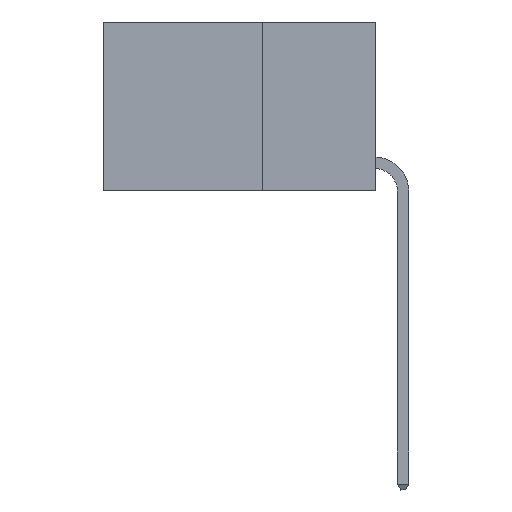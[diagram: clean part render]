
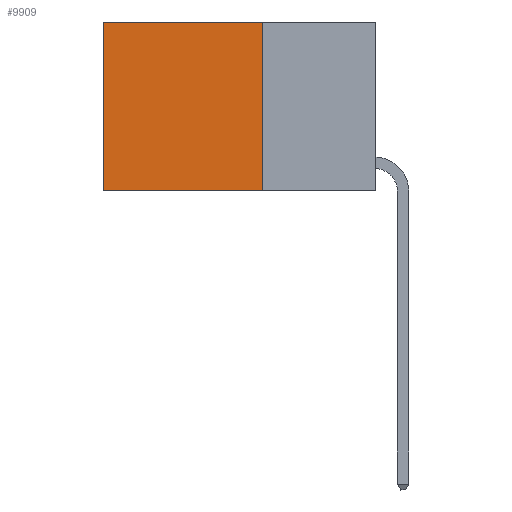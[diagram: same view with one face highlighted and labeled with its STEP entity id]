
A CAD part, left-side view. The second image highlights one B-rep face of the part: STEP entity #9909.
In plain terms, the highlighted planar face has unit normal (-1, 0, 0).
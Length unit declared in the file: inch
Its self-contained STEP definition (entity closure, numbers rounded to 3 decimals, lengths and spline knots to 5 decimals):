
#14 = ORIENTED_EDGE ( 'NONE', *, *, #6676, .F. ) ;
#56 = DIRECTION ( 'NONE',  ( 0., 1., 0. ) ) ;
#680 = LINE ( 'NONE', #17780, #11102 ) ;
#866 = DIRECTION ( 'NONE',  ( 1., 0., 0. ) ) ;
#932 = VECTOR ( 'NONE', #56, 39.37008 ) ;
#1865 = VERTEX_POINT ( 'NONE', #22350 ) ;
#2255 = CARTESIAN_POINT ( 'NONE',  ( 0.2625, 0.25, -0.37 ) ) ;
#2408 = VECTOR ( 'NONE', #11072, 39.37008 ) ;
#3258 = PLANE ( 'NONE',  #25943 ) ;
#4280 = CARTESIAN_POINT ( 'NONE',  ( 0.2625, 0.25, 0. ) ) ;
#4566 = CARTESIAN_POINT ( 'NONE',  ( 0.2625, 0.25, 0. ) ) ;
#4712 = VERTEX_POINT ( 'NONE', #4566 ) ;
#6676 = EDGE_CURVE ( 'NONE', #11924, #1865, #15924, .T. ) ;
#8476 = DIRECTION ( 'NONE',  ( 0., 0., -1. ) ) ;
#9704 = FACE_OUTER_BOUND ( 'NONE', #10836, .T. ) ;
#9909 = ADVANCED_FACE ( 'NONE', ( #9704 ), #3258, .F. ) ;
#10712 = LINE ( 'NONE', #25705, #13535 ) ;
#10836 = EDGE_LOOP ( 'NONE', ( #19209, #14, #17049, #22264 ) ) ;
#11072 = DIRECTION ( 'NONE',  ( 0., 1., 0. ) ) ;
#11102 = VECTOR ( 'NONE', #22069, 39.37008 ) ;
#11924 = VERTEX_POINT ( 'NONE', #25751 ) ;
#13535 = VECTOR ( 'NONE', #8476, 39.37008 ) ;
#13536 = VERTEX_POINT ( 'NONE', #20876 ) ;
#15880 = EDGE_CURVE ( 'NONE', #13536, #1865, #680, .T. ) ;
#15924 = LINE ( 'NONE', #2255, #2408 ) ;
#17049 = ORIENTED_EDGE ( 'NONE', *, *, #22934, .F. ) ;
#17780 = CARTESIAN_POINT ( 'NONE',  ( 0.2625, 0.6, 0. ) ) ;
#18230 = CARTESIAN_POINT ( 'NONE',  ( 0.2625, 0.25, 0. ) ) ;
#19209 = ORIENTED_EDGE ( 'NONE', *, *, #15880, .T. ) ;
#20053 = EDGE_CURVE ( 'NONE', #4712, #13536, #23381, .T. ) ;
#20140 = DIRECTION ( 'NONE',  ( 0., 0., -1. ) ) ;
#20876 = CARTESIAN_POINT ( 'NONE',  ( 0.2625, 0.6, 0. ) ) ;
#22069 = DIRECTION ( 'NONE',  ( 0., 0., -1. ) ) ;
#22264 = ORIENTED_EDGE ( 'NONE', *, *, #20053, .T. ) ;
#22350 = CARTESIAN_POINT ( 'NONE',  ( 0.2625, 0.6, -0.37 ) ) ;
#22934 = EDGE_CURVE ( 'NONE', #4712, #11924, #10712, .T. ) ;
#23381 = LINE ( 'NONE', #4280, #932 ) ;
#25705 = CARTESIAN_POINT ( 'NONE',  ( 0.2625, 0.25, 0. ) ) ;
#25751 = CARTESIAN_POINT ( 'NONE',  ( 0.2625, 0.25, -0.37 ) ) ;
#25943 = AXIS2_PLACEMENT_3D ( 'NONE', #18230, #866, #20140 ) ;
